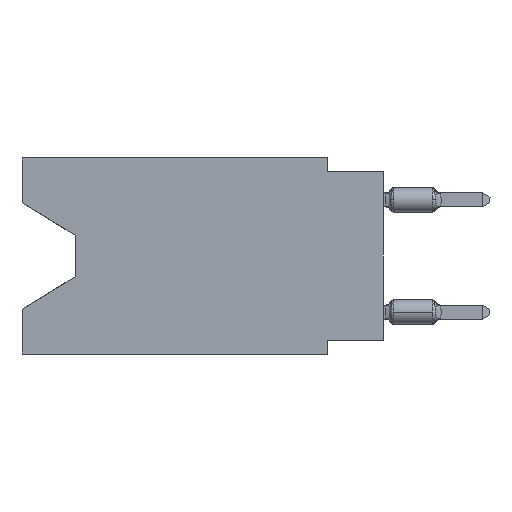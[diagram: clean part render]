
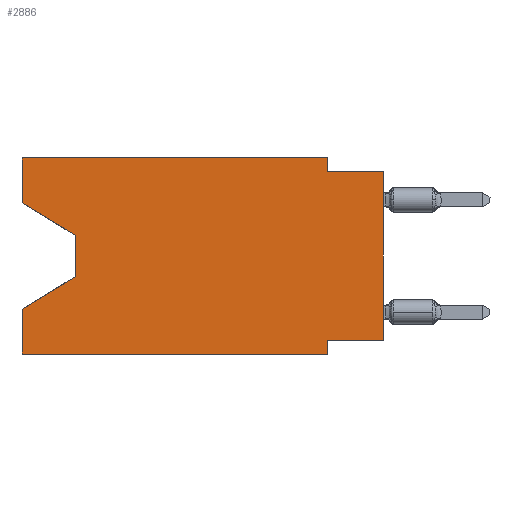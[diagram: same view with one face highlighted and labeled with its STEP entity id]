
A CAD part, left-side view. The second image highlights one B-rep face of the part: STEP entity #2886.
In plain terms, the highlighted planar face has unit normal (-1, 0, 0).
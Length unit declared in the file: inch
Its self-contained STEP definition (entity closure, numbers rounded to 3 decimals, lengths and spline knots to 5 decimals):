
#159 = ORIENTED_EDGE ( 'NONE', *, *, #9891, .F. ) ;
#167 = CARTESIAN_POINT ( 'NONE',  ( 0., 0.645, -0.26975 ) ) ;
#434 = EDGE_CURVE ( 'NONE', #3590, #8614, #8362, .T. ) ;
#682 = VECTOR ( 'NONE', #22460, 39.37008 ) ;
#983 = CARTESIAN_POINT ( 'NONE',  ( 0., 0., -0.325 ) ) ;
#1067 = CARTESIAN_POINT ( 'NONE',  ( 0., 0., -0.325 ) ) ;
#1397 = VERTEX_POINT ( 'NONE', #13078 ) ;
#1403 = EDGE_CURVE ( 'NONE', #4421, #4781, #9038, .T. ) ;
#1446 = ORIENTED_EDGE ( 'NONE', *, *, #2453, .T. ) ;
#1757 = LINE ( 'NONE', #6056, #682 ) ;
#1986 = LINE ( 'NONE', #8428, #17341 ) ;
#2003 = CARTESIAN_POINT ( 'NONE',  ( 0., 0.645, 0. ) ) ;
#2453 = EDGE_CURVE ( 'NONE', #6373, #1397, #19464, .T. ) ;
#2886 = ADVANCED_FACE ( 'NONE', ( #23212 ), #19781, .F. ) ;
#3006 = DIRECTION ( 'NONE',  ( 0., 0., 1. ) ) ;
#3590 = VERTEX_POINT ( 'NONE', #983 ) ;
#3947 = ORIENTED_EDGE ( 'NONE', *, *, #8957, .T. ) ;
#4138 = CARTESIAN_POINT ( 'NONE',  ( 0., 0.1, 0. ) ) ;
#4200 = CARTESIAN_POINT ( 'NONE',  ( 0., 0., 0. ) ) ;
#4421 = VERTEX_POINT ( 'NONE', #21497 ) ;
#4539 = VERTEX_POINT ( 'NONE', #17722 ) ;
#4781 = VERTEX_POINT ( 'NONE', #19015 ) ;
#4796 = CARTESIAN_POINT ( 'NONE',  ( 0., 0.645, -0.08025 ) ) ;
#4925 = ORIENTED_EDGE ( 'NONE', *, *, #13383, .F. ) ;
#5499 = VECTOR ( 'NONE', #13589, 39.37008 ) ;
#6056 = CARTESIAN_POINT ( 'NONE',  ( 0., 0.55, -0.212 ) ) ;
#6373 = VERTEX_POINT ( 'NONE', #6748 ) ;
#6617 = ORIENTED_EDGE ( 'NONE', *, *, #1403, .F. ) ;
#6748 = CARTESIAN_POINT ( 'NONE',  ( 0., 0.645, -0.35 ) ) ;
#6791 = LINE ( 'NONE', #15009, #17892 ) ;
#7027 = LINE ( 'NONE', #19136, #12369 ) ;
#7369 = ORIENTED_EDGE ( 'NONE', *, *, #434, .T. ) ;
#7490 = LINE ( 'NONE', #22147, #16704 ) ;
#7534 = EDGE_CURVE ( 'NONE', #4539, #8337, #1757, .T. ) ;
#7604 = VECTOR ( 'NONE', #15431, 39.37008 ) ;
#8337 = VERTEX_POINT ( 'NONE', #167 ) ;
#8362 = LINE ( 'NONE', #4200, #8526 ) ;
#8428 = CARTESIAN_POINT ( 'NONE',  ( 0., 0.1, -0.35 ) ) ;
#8526 = VECTOR ( 'NONE', #16298, 39.37008 ) ;
#8614 = VERTEX_POINT ( 'NONE', #20301 ) ;
#8957 = EDGE_CURVE ( 'NONE', #25175, #24896, #18940, .T. ) ;
#9038 = LINE ( 'NONE', #4138, #25339 ) ;
#9891 = EDGE_CURVE ( 'NONE', #3590, #16793, #25837, .T. ) ;
#10414 = EDGE_CURVE ( 'NONE', #24896, #4539, #7490, .T. ) ;
#10573 = DIRECTION ( 'NONE',  ( 0., 0., -1. ) ) ;
#10662 = CARTESIAN_POINT ( 'NONE',  ( 0., 0.645, -0.08025 ) ) ;
#11235 = CARTESIAN_POINT ( 'NONE',  ( 0., 0.645, 0. ) ) ;
#11659 = CARTESIAN_POINT ( 'NONE',  ( 0., 0.645, 0. ) ) ;
#11787 = DIRECTION ( 'NONE',  ( 0., 0., -1. ) ) ;
#12206 = AXIS2_PLACEMENT_3D ( 'NONE', #2003, #14373, #15881 ) ;
#12224 = VECTOR ( 'NONE', #23360, 39.37008 ) ;
#12369 = VECTOR ( 'NONE', #3006, 39.37008 ) ;
#12448 = EDGE_CURVE ( 'NONE', #6373, #8337, #7027, .T. ) ;
#12699 = VECTOR ( 'NONE', #19446, 39.37008 ) ;
#13078 = CARTESIAN_POINT ( 'NONE',  ( 0., 0.1, -0.35 ) ) ;
#13268 = LINE ( 'NONE', #11235, #12699 ) ;
#13383 = EDGE_CURVE ( 'NONE', #25175, #26160, #13268, .T. ) ;
#13589 = DIRECTION ( 'NONE',  ( 0., 1., 0. ) ) ;
#13621 = ORIENTED_EDGE ( 'NONE', *, *, #15862, .F. ) ;
#13703 = ORIENTED_EDGE ( 'NONE', *, *, #16268, .F. ) ;
#14373 = DIRECTION ( 'NONE',  ( 1., 0., 0. ) ) ;
#14631 = DIRECTION ( 'NONE',  ( 0., 0., -1. ) ) ;
#15009 = CARTESIAN_POINT ( 'NONE',  ( 0., 0., -0.025 ) ) ;
#15431 = DIRECTION ( 'NONE',  ( 0., -1., 0. ) ) ;
#15862 = EDGE_CURVE ( 'NONE', #4781, #8614, #6791, .T. ) ;
#15881 = DIRECTION ( 'NONE',  ( 0., 0., -1. ) ) ;
#16268 = EDGE_CURVE ( 'NONE', #26160, #4421, #19329, .T. ) ;
#16298 = DIRECTION ( 'NONE',  ( 0., 0., 1. ) ) ;
#16480 = ORIENTED_EDGE ( 'NONE', *, *, #10414, .T. ) ;
#16704 = VECTOR ( 'NONE', #11787, 39.37008 ) ;
#16793 = VERTEX_POINT ( 'NONE', #22879 ) ;
#17341 = VECTOR ( 'NONE', #10573, 39.37008 ) ;
#17482 = CARTESIAN_POINT ( 'NONE',  ( 0., 0.645, 0. ) ) ;
#17722 = CARTESIAN_POINT ( 'NONE',  ( 0., 0.55, -0.212 ) ) ;
#17892 = VECTOR ( 'NONE', #19303, 39.37008 ) ;
#18584 = ORIENTED_EDGE ( 'NONE', *, *, #21395, .F. ) ;
#18940 = LINE ( 'NONE', #4796, #21878 ) ;
#19015 = CARTESIAN_POINT ( 'NONE',  ( 0., 0.1, -0.025 ) ) ;
#19136 = CARTESIAN_POINT ( 'NONE',  ( 0., 0.645, 0. ) ) ;
#19303 = DIRECTION ( 'NONE',  ( 0., -1., 0. ) ) ;
#19329 = LINE ( 'NONE', #11659, #7604 ) ;
#19446 = DIRECTION ( 'NONE',  ( 0., 0., 1. ) ) ;
#19464 = LINE ( 'NONE', #19602, #12224 ) ;
#19547 = ORIENTED_EDGE ( 'NONE', *, *, #7534, .T. ) ;
#19602 = CARTESIAN_POINT ( 'NONE',  ( 0., 0.645, -0.35 ) ) ;
#19781 = PLANE ( 'NONE',  #12206 ) ;
#20301 = CARTESIAN_POINT ( 'NONE',  ( 0., 0., -0.025 ) ) ;
#20668 = CARTESIAN_POINT ( 'NONE',  ( 0., 0.55, -0.138 ) ) ;
#21395 = EDGE_CURVE ( 'NONE', #16793, #1397, #1986, .T. ) ;
#21497 = CARTESIAN_POINT ( 'NONE',  ( 0., 0.1, 0. ) ) ;
#21878 = VECTOR ( 'NONE', #23497, 39.37008 ) ;
#22147 = CARTESIAN_POINT ( 'NONE',  ( 0., 0.55, -0.138 ) ) ;
#22210 = EDGE_LOOP ( 'NONE', ( #3947, #16480, #19547, #22445, #1446, #18584, #159, #7369, #13621, #6617, #13703, #4925 ) ) ;
#22445 = ORIENTED_EDGE ( 'NONE', *, *, #12448, .F. ) ;
#22460 = DIRECTION ( 'NONE',  ( 0., 0.855, -0.519 ) ) ;
#22879 = CARTESIAN_POINT ( 'NONE',  ( 0., 0.1, -0.325 ) ) ;
#23212 = FACE_OUTER_BOUND ( 'NONE', #22210, .T. ) ;
#23360 = DIRECTION ( 'NONE',  ( 0., -1., 0. ) ) ;
#23497 = DIRECTION ( 'NONE',  ( 0., -0.855, -0.519 ) ) ;
#24896 = VERTEX_POINT ( 'NONE', #20668 ) ;
#25175 = VERTEX_POINT ( 'NONE', #10662 ) ;
#25339 = VECTOR ( 'NONE', #14631, 39.37008 ) ;
#25837 = LINE ( 'NONE', #1067, #5499 ) ;
#26160 = VERTEX_POINT ( 'NONE', #17482 ) ;
